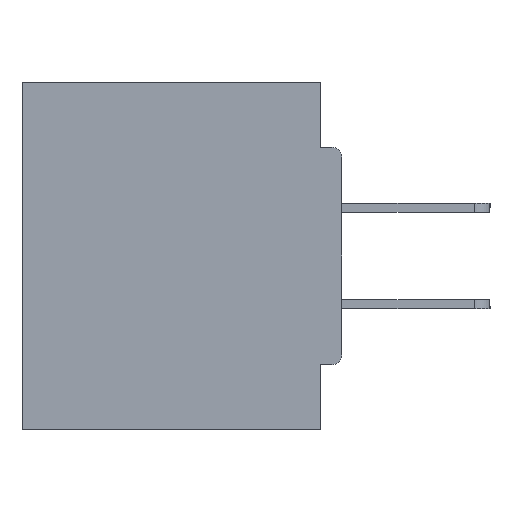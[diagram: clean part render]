
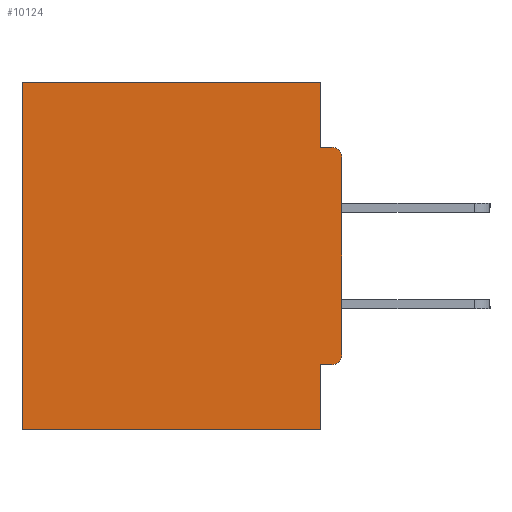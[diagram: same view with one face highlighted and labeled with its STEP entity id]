
A CAD part, left-side view. The second image highlights one B-rep face of the part: STEP entity #10124.
In plain terms, the highlighted planar face has unit normal (-1, 0, 0).
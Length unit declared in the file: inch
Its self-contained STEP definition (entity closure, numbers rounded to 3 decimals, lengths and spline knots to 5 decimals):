
#295 = CARTESIAN_POINT ( 'NONE',  ( 0.298, 0.015, -0.1085 ) ) ;
#627 = ORIENTED_EDGE ( 'NONE', *, *, #3918, .T. ) ;
#837 = VECTOR ( 'NONE', #3308, 39.37008 ) ;
#841 = EDGE_LOOP ( 'NONE', ( #22075, #20205, #24446, #5291, #627, #28560, #6756, #4287, #2144, #15618 ) ) ;
#1314 = LINE ( 'NONE', #10555, #23374 ) ;
#1764 = EDGE_CURVE ( 'NONE', #31075, #25057, #18481, .T. ) ;
#2144 = ORIENTED_EDGE ( 'NONE', *, *, #31068, .T. ) ;
#2777 = AXIS2_PLACEMENT_3D ( 'NONE', #6867, #20150, #30780 ) ;
#2985 = AXIS2_PLACEMENT_3D ( 'NONE', #295, #16496, #13474 ) ;
#3067 = CARTESIAN_POINT ( 'NONE',  ( 0.298, 0., -0.0935 ) ) ;
#3308 = DIRECTION ( 'NONE',  ( 0., -1., 0. ) ) ;
#3359 = DIRECTION ( 'NONE',  ( 0., 1., 0. ) ) ;
#3918 = EDGE_CURVE ( 'NONE', #9967, #9608, #16192, .T. ) ;
#3963 = EDGE_CURVE ( 'NONE', #12391, #25845, #10800, .T. ) ;
#3984 = CARTESIAN_POINT ( 'NONE',  ( 0.298, 0.031, -0.5 ) ) ;
#4287 = ORIENTED_EDGE ( 'NONE', *, *, #1764, .F. ) ;
#4497 = EDGE_CURVE ( 'NONE', #12391, #33665, #17852, .T. ) ;
#5291 = ORIENTED_EDGE ( 'NONE', *, *, #29375, .T. ) ;
#5875 = LINE ( 'NONE', #3984, #33345 ) ;
#6756 = ORIENTED_EDGE ( 'NONE', *, *, #8544, .F. ) ;
#6867 = CARTESIAN_POINT ( 'NONE',  ( 0.298, 0.015, -0.3915 ) ) ;
#8237 = DIRECTION ( 'NONE',  ( 0., 0., -1. ) ) ;
#8544 = EDGE_CURVE ( 'NONE', #25057, #25927, #5875, .T. ) ;
#9250 = PLANE ( 'NONE',  #13397 ) ;
#9483 = LINE ( 'NONE', #19441, #24420 ) ;
#9608 = VERTEX_POINT ( 'NONE', #13821 ) ;
#9967 = VERTEX_POINT ( 'NONE', #11792 ) ;
#10124 = ADVANCED_FACE ( 'NONE', ( #13637 ), #9250, .F. ) ;
#10555 = CARTESIAN_POINT ( 'NONE',  ( 0.298, 0., 0. ) ) ;
#10800 = CIRCLE ( 'NONE', #2985, 0.015 ) ;
#11792 = CARTESIAN_POINT ( 'NONE',  ( 0.298, 0.46, 0. ) ) ;
#11908 = DIRECTION ( 'NONE',  ( 1., 0., 0. ) ) ;
#12391 = VERTEX_POINT ( 'NONE', #28554 ) ;
#12622 = VECTOR ( 'NONE', #30769, 39.37008 ) ;
#13096 = DIRECTION ( 'NONE',  ( 0., 0., -1. ) ) ;
#13397 = AXIS2_PLACEMENT_3D ( 'NONE', #27796, #11908, #14588 ) ;
#13474 = DIRECTION ( 'NONE',  ( 0., 0., -1. ) ) ;
#13637 = FACE_OUTER_BOUND ( 'NONE', #841, .T. ) ;
#13821 = CARTESIAN_POINT ( 'NONE',  ( 0.298, 0.46, -0.5 ) ) ;
#14240 = VERTEX_POINT ( 'NONE', #33861 ) ;
#14588 = DIRECTION ( 'NONE',  ( 0., 0., -1. ) ) ;
#14851 = DIRECTION ( 'NONE',  ( 0., 0., -1. ) ) ;
#15040 = EDGE_CURVE ( 'NONE', #25927, #9608, #9483, .T. ) ;
#15618 = ORIENTED_EDGE ( 'NONE', *, *, #4497, .F. ) ;
#15779 = CARTESIAN_POINT ( 'NONE',  ( 0.298, 0., 0. ) ) ;
#16192 = LINE ( 'NONE', #21390, #20791 ) ;
#16496 = DIRECTION ( 'NONE',  ( -1., 0., 0. ) ) ;
#17647 = CARTESIAN_POINT ( 'NONE',  ( 0.298, 0.031, -0.5 ) ) ;
#17852 = LINE ( 'NONE', #15779, #29032 ) ;
#18213 = VERTEX_POINT ( 'NONE', #33671 ) ;
#18481 = LINE ( 'NONE', #26340, #12622 ) ;
#18638 = CARTESIAN_POINT ( 'NONE',  ( 0.298, 0.031, -0.5 ) ) ;
#19441 = CARTESIAN_POINT ( 'NONE',  ( 0.298, 0., -0.5 ) ) ;
#19973 = DIRECTION ( 'NONE',  ( 0., 0., -1. ) ) ;
#20150 = DIRECTION ( 'NONE',  ( -1., 0., 0. ) ) ;
#20205 = ORIENTED_EDGE ( 'NONE', *, *, #33529, .F. ) ;
#20791 = VECTOR ( 'NONE', #8237, 39.37008 ) ;
#21076 = CARTESIAN_POINT ( 'NONE',  ( 0.298, 0.015, -0.0935 ) ) ;
#21390 = CARTESIAN_POINT ( 'NONE',  ( 0.298, 0.46, 0. ) ) ;
#21869 = CIRCLE ( 'NONE', #2777, 0.015 ) ;
#22075 = ORIENTED_EDGE ( 'NONE', *, *, #3963, .T. ) ;
#22224 = VECTOR ( 'NONE', #14851, 39.37008 ) ;
#23374 = VECTOR ( 'NONE', #29211, 39.37008 ) ;
#24130 = CARTESIAN_POINT ( 'NONE',  ( 0.298, 0.031, -0.4065 ) ) ;
#24420 = VECTOR ( 'NONE', #3359, 39.37008 ) ;
#24446 = ORIENTED_EDGE ( 'NONE', *, *, #28533, .F. ) ;
#25057 = VERTEX_POINT ( 'NONE', #24130 ) ;
#25359 = CARTESIAN_POINT ( 'NONE',  ( 0.298, 0., -0.3915 ) ) ;
#25845 = VERTEX_POINT ( 'NONE', #21076 ) ;
#25927 = VERTEX_POINT ( 'NONE', #18638 ) ;
#26340 = CARTESIAN_POINT ( 'NONE',  ( 0.298, 0., -0.4065 ) ) ;
#27796 = CARTESIAN_POINT ( 'NONE',  ( 0.298, 0., 0. ) ) ;
#28094 = CARTESIAN_POINT ( 'NONE',  ( 0.298, 0.015, -0.4065 ) ) ;
#28533 = EDGE_CURVE ( 'NONE', #14240, #18213, #29256, .T. ) ;
#28554 = CARTESIAN_POINT ( 'NONE',  ( 0.298, 0., -0.1085 ) ) ;
#28560 = ORIENTED_EDGE ( 'NONE', *, *, #15040, .F. ) ;
#29032 = VECTOR ( 'NONE', #13096, 39.37008 ) ;
#29211 = DIRECTION ( 'NONE',  ( 0., 1., 0. ) ) ;
#29256 = LINE ( 'NONE', #17647, #22224 ) ;
#29375 = EDGE_CURVE ( 'NONE', #14240, #9967, #1314, .T. ) ;
#30769 = DIRECTION ( 'NONE',  ( 0., 1., 0. ) ) ;
#30780 = DIRECTION ( 'NONE',  ( 0., 0., -1. ) ) ;
#31068 = EDGE_CURVE ( 'NONE', #31075, #33665, #21869, .T. ) ;
#31075 = VERTEX_POINT ( 'NONE', #28094 ) ;
#32060 = LINE ( 'NONE', #3067, #837 ) ;
#33345 = VECTOR ( 'NONE', #19973, 39.37008 ) ;
#33529 = EDGE_CURVE ( 'NONE', #18213, #25845, #32060, .T. ) ;
#33665 = VERTEX_POINT ( 'NONE', #25359 ) ;
#33671 = CARTESIAN_POINT ( 'NONE',  ( 0.298, 0.031, -0.0935 ) ) ;
#33861 = CARTESIAN_POINT ( 'NONE',  ( 0.298, 0.031, 0. ) ) ;
